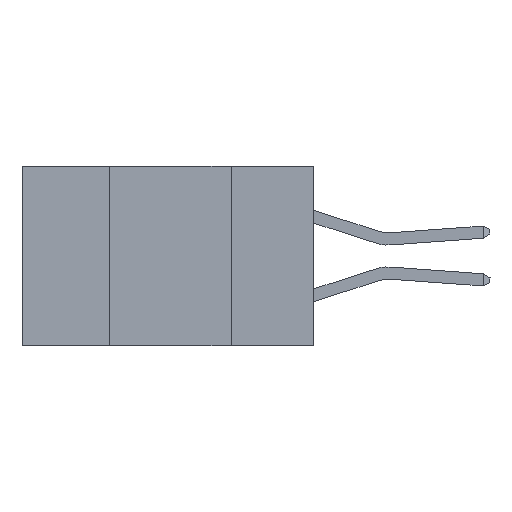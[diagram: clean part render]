
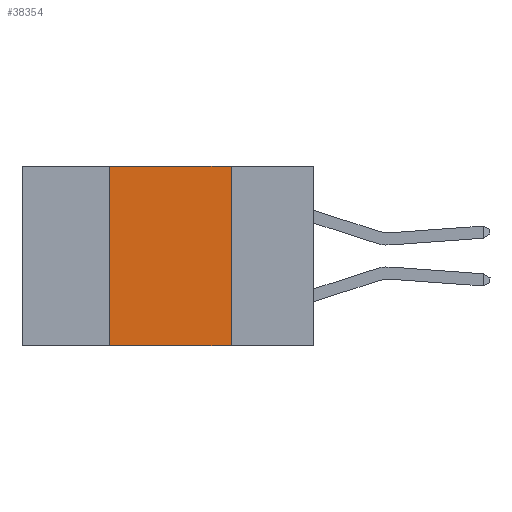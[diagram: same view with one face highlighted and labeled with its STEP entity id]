
A CAD part, left-side view. The second image highlights one B-rep face of the part: STEP entity #38354.
In plain terms, the highlighted planar face has unit normal (-1, 0, 0).
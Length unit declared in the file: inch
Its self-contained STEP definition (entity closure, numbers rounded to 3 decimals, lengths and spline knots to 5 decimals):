
#1802 = EDGE_CURVE ( 'NONE', #29119, #30538, #45423, .T. ) ;
#3562 = CARTESIAN_POINT ( 'NONE',  ( 0., 0.6, 0. ) ) ;
#3814 = EDGE_CURVE ( 'NONE', #44763, #29551, #39681, .T. ) ;
#4544 = EDGE_LOOP ( 'NONE', ( #11933, #24467, #20249, #26120 ) ) ;
#5909 = VECTOR ( 'NONE', #42381, 39.37008 ) ;
#6077 = CARTESIAN_POINT ( 'NONE',  ( 0., 0.42, -0.37 ) ) ;
#8027 = CARTESIAN_POINT ( 'NONE',  ( 0., 0.17, -0.37 ) ) ;
#10334 = DIRECTION ( 'NONE',  ( 0., 0., -1. ) ) ;
#11162 = VECTOR ( 'NONE', #30875, 39.37008 ) ;
#11933 = ORIENTED_EDGE ( 'NONE', *, *, #3814, .F. ) ;
#12234 = VECTOR ( 'NONE', #19419, 39.37008 ) ;
#12356 = CARTESIAN_POINT ( 'NONE',  ( 0., 0.6, -0.37 ) ) ;
#19419 = DIRECTION ( 'NONE',  ( 0., -1., 0. ) ) ;
#20249 = ORIENTED_EDGE ( 'NONE', *, *, #1802, .F. ) ;
#22889 = VECTOR ( 'NONE', #23242, 39.37008 ) ;
#23102 = CARTESIAN_POINT ( 'NONE',  ( 0., 0.6, 0. ) ) ;
#23242 = DIRECTION ( 'NONE',  ( 0., -1., 0. ) ) ;
#24467 = ORIENTED_EDGE ( 'NONE', *, *, #34583, .F. ) ;
#26120 = ORIENTED_EDGE ( 'NONE', *, *, #41247, .T. ) ;
#28871 = CARTESIAN_POINT ( 'NONE',  ( 0., 0.42, 0. ) ) ;
#29119 = VERTEX_POINT ( 'NONE', #6077 ) ;
#29185 = LINE ( 'NONE', #12356, #12234 ) ;
#29551 = VERTEX_POINT ( 'NONE', #8027 ) ;
#30538 = VERTEX_POINT ( 'NONE', #35148 ) ;
#30875 = DIRECTION ( 'NONE',  ( 0., 0., -1. ) ) ;
#34583 = EDGE_CURVE ( 'NONE', #30538, #44763, #39327, .T. ) ;
#35148 = CARTESIAN_POINT ( 'NONE',  ( 0., 0.42, 0. ) ) ;
#36075 = AXIS2_PLACEMENT_3D ( 'NONE', #3562, #41911, #10334 ) ;
#38221 = CARTESIAN_POINT ( 'NONE',  ( 0., 0.17, 0. ) ) ;
#38354 = ADVANCED_FACE ( 'NONE', ( #42312 ), #45295, .F. ) ;
#39327 = LINE ( 'NONE', #23102, #22889 ) ;
#39681 = LINE ( 'NONE', #38221, #11162 ) ;
#41247 = EDGE_CURVE ( 'NONE', #29119, #29551, #29185, .T. ) ;
#41911 = DIRECTION ( 'NONE',  ( 1., 0., 0. ) ) ;
#42312 = FACE_OUTER_BOUND ( 'NONE', #4544, .T. ) ;
#42381 = DIRECTION ( 'NONE',  ( 0., 0., 1. ) ) ;
#42711 = CARTESIAN_POINT ( 'NONE',  ( 0., 0.17, 0. ) ) ;
#44763 = VERTEX_POINT ( 'NONE', #42711 ) ;
#45295 = PLANE ( 'NONE',  #36075 ) ;
#45423 = LINE ( 'NONE', #28871, #5909 ) ;
